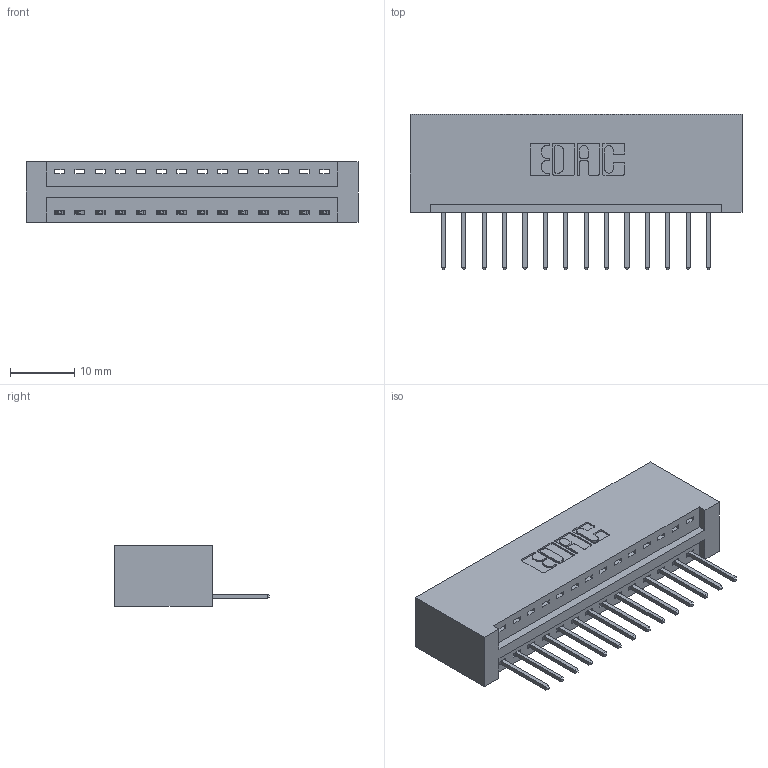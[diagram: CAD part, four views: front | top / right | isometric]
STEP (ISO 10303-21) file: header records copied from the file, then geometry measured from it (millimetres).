
FILE_DESCRIPTION (( 'STEP AP203' ), '1' );
FILE_NAME ('396-014-526-101.STEP', '2019-10-26T16:47:42', ( '' ), ( '' ), 'SwSTEP 2.0', 'SolidWorks 2016', '' );
FILE_SCHEMA (( 'CONFIG_CONTROL_DESIGN' ));
Length unit declared in the file: inch
Products named in the file (3): 345-292-001_345-293-126; 396-014-526-101; 346 Part_No Mounting Lugs
Assembly tree (15 placements, depth 2):
  396-014-526-101
    346 Part_No Mounting Lugs
    345-292-001_345-293-126  x14
Bounding box: 51.69 x 24.13 x 9.4 mm (x, y, z)
Volume: 5293.1 mm3; surface area: 6375 mm2
Topology: 15 solids, 15 shells, 926 faces, 2769 edges, 1826 vertices
Faces by surface type: plane 632, cylinder 294
Entity records: 12199 total; most frequent: CARTESIAN_POINT 2106, ORIENTED_EDGE 2054, DIRECTION 1887, EDGE_CURVE 1027, LINE 847, VECTOR 847, VERTEX_POINT 682, AXIS2_PLACEMENT_3D 520
